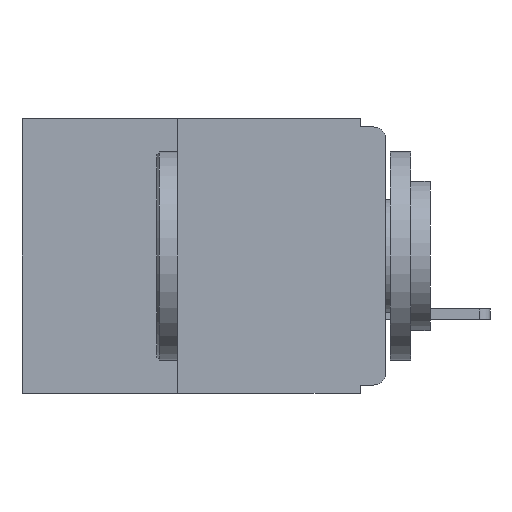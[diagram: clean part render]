
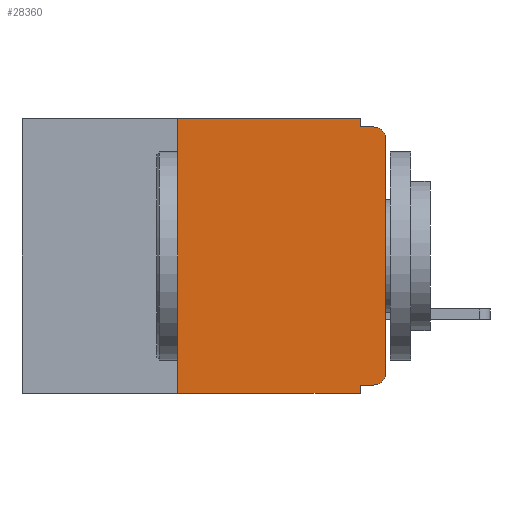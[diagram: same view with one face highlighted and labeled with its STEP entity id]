
A CAD part, left-side view. The second image highlights one B-rep face of the part: STEP entity #28360.
In plain terms, the highlighted planar face has unit normal (-1, 0, 0).
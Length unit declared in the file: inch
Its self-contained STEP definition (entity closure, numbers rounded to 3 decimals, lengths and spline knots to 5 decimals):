
#198 = VECTOR ( 'NONE', #8029, 39.37008 ) ;
#733 = EDGE_CURVE ( 'NONE', #5285, #6873, #19974, .T. ) ;
#1291 = CARTESIAN_POINT ( 'NONE',  ( 0., 0., -0.32 ) ) ;
#1893 = LINE ( 'NONE', #27902, #28879 ) ;
#2777 = ORIENTED_EDGE ( 'NONE', *, *, #23868, .F. ) ;
#2870 = LINE ( 'NONE', #5568, #15942 ) ;
#3989 = VERTEX_POINT ( 'NONE', #22097 ) ;
#4408 = LINE ( 'NONE', #1291, #24450 ) ;
#5285 = VERTEX_POINT ( 'NONE', #28733 ) ;
#5568 = CARTESIAN_POINT ( 'NONE',  ( 0., 0.437, -0.33 ) ) ;
#5652 = AXIS2_PLACEMENT_3D ( 'NONE', #24084, #19378, #11856 ) ;
#5959 = AXIS2_PLACEMENT_3D ( 'NONE', #13168, #31404, #15787 ) ;
#6520 = EDGE_CURVE ( 'NONE', #7341, #33099, #6675, .T. ) ;
#6675 = LINE ( 'NONE', #23393, #12823 ) ;
#6873 = VERTEX_POINT ( 'NONE', #17502 ) ;
#6923 = EDGE_CURVE ( 'NONE', #33099, #10966, #28357, .T. ) ;
#7015 = CARTESIAN_POINT ( 'NONE',  ( 0., 0., -0.01 ) ) ;
#7341 = VERTEX_POINT ( 'NONE', #14200 ) ;
#7456 = VECTOR ( 'NONE', #15125, 39.37008 ) ;
#7593 = CARTESIAN_POINT ( 'NONE',  ( 0., 0.25, -0.33 ) ) ;
#7659 = ORIENTED_EDGE ( 'NONE', *, *, #21240, .T. ) ;
#8029 = DIRECTION ( 'NONE',  ( 0., 0., 1. ) ) ;
#8063 = VERTEX_POINT ( 'NONE', #24091 ) ;
#8128 = ORIENTED_EDGE ( 'NONE', *, *, #6520, .F. ) ;
#8195 = DIRECTION ( 'NONE',  ( 0., -1., 0. ) ) ;
#8697 = ORIENTED_EDGE ( 'NONE', *, *, #18130, .F. ) ;
#8804 = CARTESIAN_POINT ( 'NONE',  ( 0., 0.437, 0. ) ) ;
#9653 = DIRECTION ( 'NONE',  ( 0., -1., 0. ) ) ;
#10351 = DIRECTION ( 'NONE',  ( 0., -1., 0. ) ) ;
#10966 = VERTEX_POINT ( 'NONE', #25316 ) ;
#11856 = DIRECTION ( 'NONE',  ( 0., 0., -1. ) ) ;
#12107 = LINE ( 'NONE', #14308, #30494 ) ;
#12499 = CARTESIAN_POINT ( 'NONE',  ( 0., 0.031, 0. ) ) ;
#12823 = VECTOR ( 'NONE', #10351, 39.37008 ) ;
#13168 = CARTESIAN_POINT ( 'NONE',  ( 0., 0.015, -0.305 ) ) ;
#13303 = AXIS2_PLACEMENT_3D ( 'NONE', #8804, #14183, #32423 ) ;
#13542 = VECTOR ( 'NONE', #9653, 39.37008 ) ;
#13712 = CARTESIAN_POINT ( 'NONE',  ( 0., 0.031, 0. ) ) ;
#14096 = LINE ( 'NONE', #21076, #198 ) ;
#14183 = DIRECTION ( 'NONE',  ( 1., 0., 0. ) ) ;
#14200 = CARTESIAN_POINT ( 'NONE',  ( 0., 0.25, 0. ) ) ;
#14308 = CARTESIAN_POINT ( 'NONE',  ( 0., 0.25, -0.33 ) ) ;
#14377 = LINE ( 'NONE', #7015, #13542 ) ;
#15125 = DIRECTION ( 'NONE',  ( 0., 0., -1. ) ) ;
#15787 = DIRECTION ( 'NONE',  ( 0., 0., -1. ) ) ;
#15942 = VECTOR ( 'NONE', #8195, 39.37008 ) ;
#17077 = ORIENTED_EDGE ( 'NONE', *, *, #6923, .F. ) ;
#17502 = CARTESIAN_POINT ( 'NONE',  ( 0., 0.015, -0.01 ) ) ;
#18130 = EDGE_CURVE ( 'NONE', #3989, #27485, #4408, .T. ) ;
#18317 = CARTESIAN_POINT ( 'NONE',  ( 0., 0.031, -0.32 ) ) ;
#19378 = DIRECTION ( 'NONE',  ( -1., 0., 0. ) ) ;
#19663 = DIRECTION ( 'NONE',  ( 0., 0., 1. ) ) ;
#19769 = CARTESIAN_POINT ( 'NONE',  ( 0., 0., -0.305 ) ) ;
#19974 = CIRCLE ( 'NONE', #5652, 0.015 ) ;
#21076 = CARTESIAN_POINT ( 'NONE',  ( 0., 0., 0. ) ) ;
#21240 = EDGE_CURVE ( 'NONE', #28431, #5285, #14096, .T. ) ;
#22042 = ORIENTED_EDGE ( 'NONE', *, *, #733, .T. ) ;
#22097 = CARTESIAN_POINT ( 'NONE',  ( 0., 0.015, -0.32 ) ) ;
#22830 = EDGE_CURVE ( 'NONE', #3989, #28431, #31125, .T. ) ;
#23393 = CARTESIAN_POINT ( 'NONE',  ( 0., 0.437, 0. ) ) ;
#23792 = ORIENTED_EDGE ( 'NONE', *, *, #26890, .F. ) ;
#23868 = EDGE_CURVE ( 'NONE', #10966, #6873, #14377, .T. ) ;
#24008 = EDGE_LOOP ( 'NONE', ( #7659, #22042, #2777, #17077, #8128, #24120, #28294, #23792, #8697, #31175 ) ) ;
#24084 = CARTESIAN_POINT ( 'NONE',  ( 0., 0.015, -0.025 ) ) ;
#24091 = CARTESIAN_POINT ( 'NONE',  ( 0., 0.031, -0.33 ) ) ;
#24120 = ORIENTED_EDGE ( 'NONE', *, *, #26801, .F. ) ;
#24450 = VECTOR ( 'NONE', #27352, 39.37008 ) ;
#25093 = FACE_OUTER_BOUND ( 'NONE', #24008, .T. ) ;
#25316 = CARTESIAN_POINT ( 'NONE',  ( 0., 0.031, -0.01 ) ) ;
#26801 = EDGE_CURVE ( 'NONE', #32535, #7341, #12107, .T. ) ;
#26890 = EDGE_CURVE ( 'NONE', #27485, #8063, #1893, .T. ) ;
#27226 = PLANE ( 'NONE',  #13303 ) ;
#27352 = DIRECTION ( 'NONE',  ( 0., 1., 0. ) ) ;
#27485 = VERTEX_POINT ( 'NONE', #18317 ) ;
#27902 = CARTESIAN_POINT ( 'NONE',  ( 0., 0.031, -0.33 ) ) ;
#28294 = ORIENTED_EDGE ( 'NONE', *, *, #30320, .T. ) ;
#28357 = LINE ( 'NONE', #12499, #7456 ) ;
#28360 = ADVANCED_FACE ( 'NONE', ( #25093 ), #27226, .F. ) ;
#28431 = VERTEX_POINT ( 'NONE', #19769 ) ;
#28733 = CARTESIAN_POINT ( 'NONE',  ( 0., 0., -0.025 ) ) ;
#28879 = VECTOR ( 'NONE', #33097, 39.37008 ) ;
#30320 = EDGE_CURVE ( 'NONE', #32535, #8063, #2870, .T. ) ;
#30494 = VECTOR ( 'NONE', #19663, 39.37008 ) ;
#31125 = CIRCLE ( 'NONE', #5959, 0.015 ) ;
#31175 = ORIENTED_EDGE ( 'NONE', *, *, #22830, .T. ) ;
#31404 = DIRECTION ( 'NONE',  ( -1., 0., 0. ) ) ;
#32423 = DIRECTION ( 'NONE',  ( 0., 0., -1. ) ) ;
#32535 = VERTEX_POINT ( 'NONE', #7593 ) ;
#33097 = DIRECTION ( 'NONE',  ( 0., 0., -1. ) ) ;
#33099 = VERTEX_POINT ( 'NONE', #13712 ) ;
